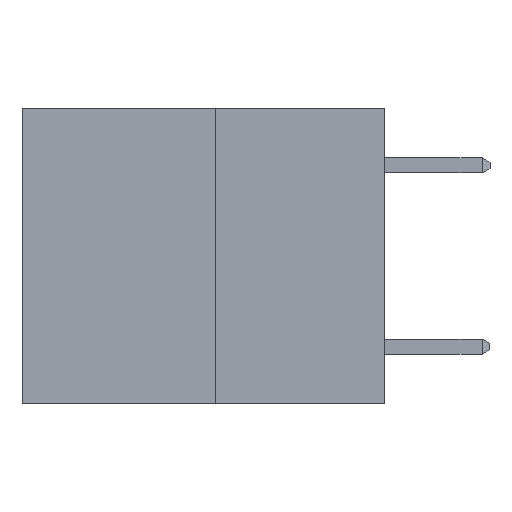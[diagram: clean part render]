
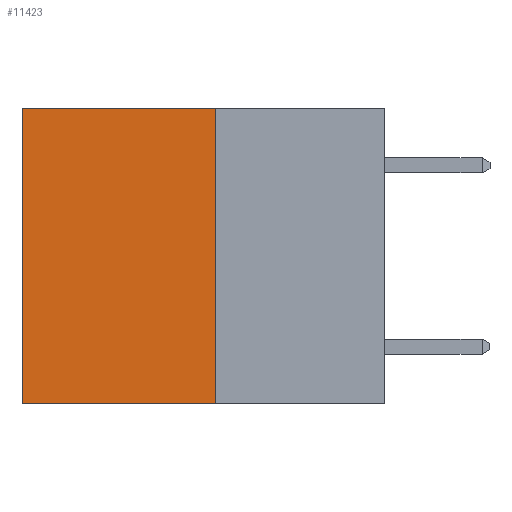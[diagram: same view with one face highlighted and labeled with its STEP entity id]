
A CAD part, left-side view. The second image highlights one B-rep face of the part: STEP entity #11423.
In plain terms, the highlighted planar face has unit normal (-1, 0, 0).
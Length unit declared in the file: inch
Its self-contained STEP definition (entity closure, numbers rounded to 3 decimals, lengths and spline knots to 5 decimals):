
#346 = VECTOR ( 'NONE', #11250, 39.37008 ) ;
#938 = CARTESIAN_POINT ( 'NONE',  ( 0.3165, 0.28, -0.49 ) ) ;
#1086 = CARTESIAN_POINT ( 'NONE',  ( 0.3165, 0.28, 0. ) ) ;
#1179 = VECTOR ( 'NONE', #6571, 39.37008 ) ;
#1207 = LINE ( 'NONE', #10104, #9433 ) ;
#1753 = DIRECTION ( 'NONE',  ( 0., 0., -1. ) ) ;
#1862 = CARTESIAN_POINT ( 'NONE',  ( 0.3165, 0.28, -0.49 ) ) ;
#2012 = ORIENTED_EDGE ( 'NONE', *, *, #12274, .T. ) ;
#3167 = AXIS2_PLACEMENT_3D ( 'NONE', #1862, #8640, #1753 ) ;
#4196 = LINE ( 'NONE', #938, #1179 ) ;
#4360 = LINE ( 'NONE', #11540, #5592 ) ;
#4727 = EDGE_CURVE ( 'NONE', #12706, #10710, #4196, .T. ) ;
#4963 = CARTESIAN_POINT ( 'NONE',  ( 0.3165, 0.6, 0. ) ) ;
#5397 = DIRECTION ( 'NONE',  ( 0., 0., -1. ) ) ;
#5484 = EDGE_CURVE ( 'NONE', #6029, #12706, #4360, .T. ) ;
#5592 = VECTOR ( 'NONE', #12388, 39.37008 ) ;
#5897 = CARTESIAN_POINT ( 'NONE',  ( 0.3165, 0.28, 0. ) ) ;
#6029 = VERTEX_POINT ( 'NONE', #5897 ) ;
#6322 = FACE_OUTER_BOUND ( 'NONE', #12036, .T. ) ;
#6377 = PLANE ( 'NONE',  #3167 ) ;
#6442 = CARTESIAN_POINT ( 'NONE',  ( 0.3165, 0.28, -0.49 ) ) ;
#6571 = DIRECTION ( 'NONE',  ( 0., 1., 0. ) ) ;
#6606 = ORIENTED_EDGE ( 'NONE', *, *, #4727, .F. ) ;
#6693 = CARTESIAN_POINT ( 'NONE',  ( 0.3165, 0.6, -0.49 ) ) ;
#7391 = ORIENTED_EDGE ( 'NONE', *, *, #5484, .F. ) ;
#8640 = DIRECTION ( 'NONE',  ( 1., 0., 0. ) ) ;
#9022 = EDGE_CURVE ( 'NONE', #6029, #12096, #9450, .T. ) ;
#9433 = VECTOR ( 'NONE', #5397, 39.37008 ) ;
#9450 = LINE ( 'NONE', #1086, #346 ) ;
#9785 = ORIENTED_EDGE ( 'NONE', *, *, #9022, .T. ) ;
#10104 = CARTESIAN_POINT ( 'NONE',  ( 0.3165, 0.6, -0.49 ) ) ;
#10710 = VERTEX_POINT ( 'NONE', #6693 ) ;
#11250 = DIRECTION ( 'NONE',  ( 0., 1., 0. ) ) ;
#11423 = ADVANCED_FACE ( 'NONE', ( #6322 ), #6377, .F. ) ;
#11540 = CARTESIAN_POINT ( 'NONE',  ( 0.3165, 0.28, -0.49 ) ) ;
#12036 = EDGE_LOOP ( 'NONE', ( #2012, #6606, #7391, #9785 ) ) ;
#12096 = VERTEX_POINT ( 'NONE', #4963 ) ;
#12274 = EDGE_CURVE ( 'NONE', #12096, #10710, #1207, .T. ) ;
#12388 = DIRECTION ( 'NONE',  ( 0., 0., -1. ) ) ;
#12706 = VERTEX_POINT ( 'NONE', #6442 ) ;
